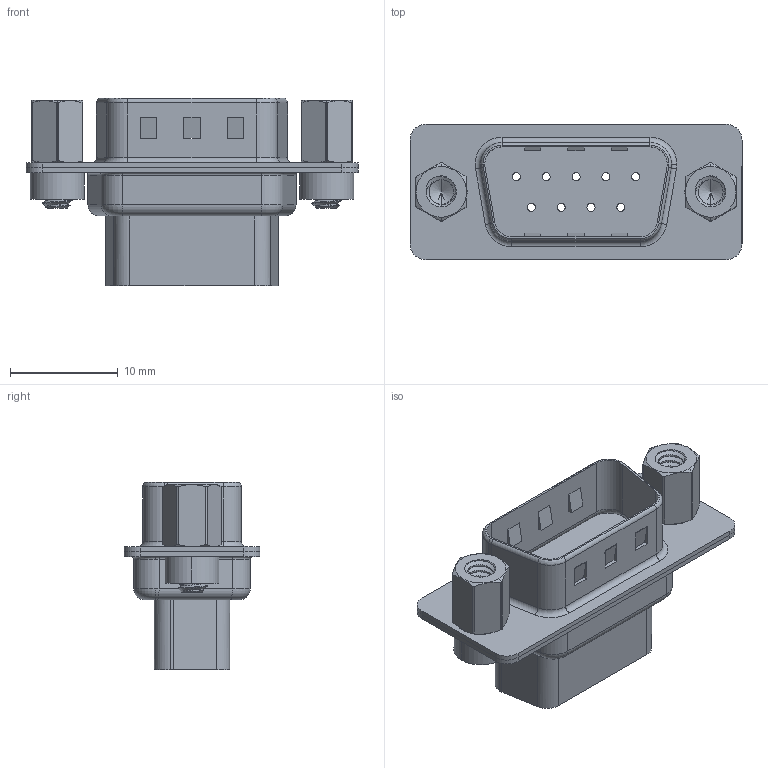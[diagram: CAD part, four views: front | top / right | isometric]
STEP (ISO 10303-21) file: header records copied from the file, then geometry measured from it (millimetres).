
FILE_DESCRIPTION (( 'STEP AP203' ), '1' );
FILE_NAME ('627-009-010-043.STEP', '2020-07-15T20:14:27', ( '' ), ( '' ), 'SwSTEP 2.0', 'SolidWorks 2020', '' );
FILE_SCHEMA (( 'CONFIG_CONTROL_DESIGN' ));
Length unit declared in the file: millimetre
Products named in the file (6): 627 Shell Rear_09 Contacts; 627-009-010-043; 627 4-40 Threaded Rivet; 627 Housing_09 HP; 627 Shell Front_09 Contacts; 627 4-40 Hex Standoff
Assembly tree (7 placements, depth 2):
  627-009-010-043
    627 Housing_09 HP
    627 Shell Front_09 Contacts
    627 Shell Rear_09 Contacts
    627 4-40 Threaded Rivet  x2
    627 4-40 Hex Standoff  x2
Bounding box: 30.8 x 12.6 x 17.4 mm (x, y, z)
Volume: 1873.9 mm3; surface area: 4033.9 mm2
Topology: 7 solids, 7 shells, 498 faces, 1257 edges, 802 vertices
Faces by surface type: cylinder 253, plane 147, torus 50, cone 30, bspline 18
Entity records: 16853 total; most frequent: CARTESIAN_POINT 6465, DIRECTION 2089, ORIENTED_EDGE 2010, EDGE_CURVE 1005, AXIS2_PLACEMENT_3D 815, VERTEX_POINT 640, EDGE_LOOP 477, VECTOR 459
